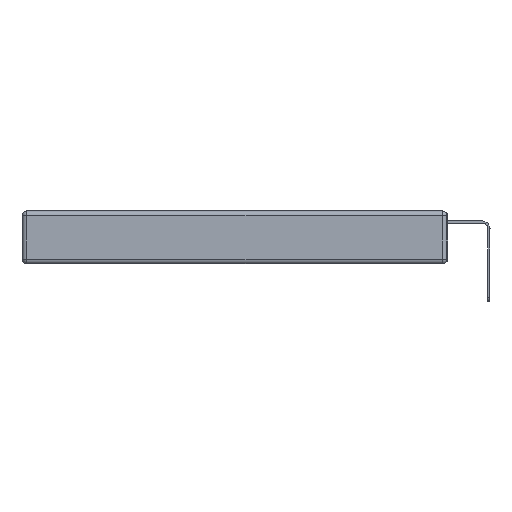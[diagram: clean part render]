
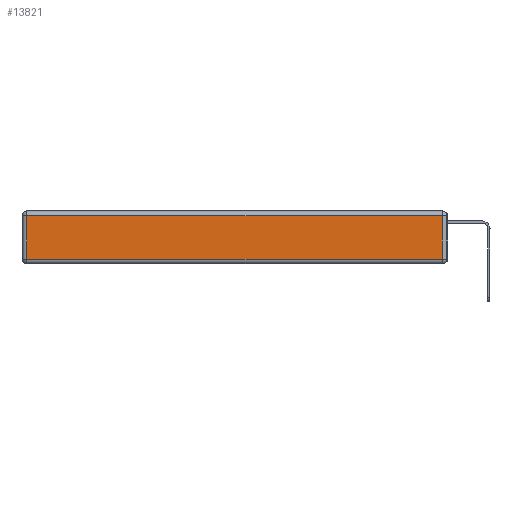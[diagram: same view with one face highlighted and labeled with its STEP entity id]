
A CAD part, left-side view. The second image highlights one B-rep face of the part: STEP entity #13821.
In plain terms, the highlighted planar face has unit normal (-1, 0, 0).
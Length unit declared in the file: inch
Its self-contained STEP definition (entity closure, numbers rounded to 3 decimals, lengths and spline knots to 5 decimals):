
#285 = CARTESIAN_POINT ( 'NONE',  ( 0., 2.72, -0.313 ) ) ;
#615 = DIRECTION ( 'NONE',  ( -1., 0., 0. ) ) ;
#757 = CARTESIAN_POINT ( 'NONE',  ( 0., 0., -0.343 ) ) ;
#773 = CARTESIAN_POINT ( 'NONE',  ( 0., 0.03, -0.03 ) ) ;
#1313 = EDGE_CURVE ( 'NONE', #16355, #19260, #4810, .T. ) ;
#2608 = LINE ( 'NONE', #7543, #11050 ) ;
#2782 = DIRECTION ( 'NONE',  ( 0., 1., 0. ) ) ;
#2871 = EDGE_LOOP ( 'NONE', ( #18262, #4706, #10884, #19595 ) ) ;
#4153 = EDGE_CURVE ( 'NONE', #19260, #10068, #19310, .T. ) ;
#4437 = CARTESIAN_POINT ( 'NONE',  ( 0., 2.72, -0.343 ) ) ;
#4706 = ORIENTED_EDGE ( 'NONE', *, *, #9290, .T. ) ;
#4810 = LINE ( 'NONE', #4437, #19940 ) ;
#7157 = CARTESIAN_POINT ( 'NONE',  ( 0., 2.72, -0.03 ) ) ;
#7543 = CARTESIAN_POINT ( 'NONE',  ( 0., 2.75, -0.03 ) ) ;
#7978 = VECTOR ( 'NONE', #19165, 39.37008 ) ;
#8050 = EDGE_CURVE ( 'NONE', #17491, #16355, #2608, .T. ) ;
#8529 = FACE_OUTER_BOUND ( 'NONE', #2871, .T. ) ;
#8962 = VECTOR ( 'NONE', #9070, 39.37008 ) ;
#9070 = DIRECTION ( 'NONE',  ( 0., 0., 1. ) ) ;
#9113 = DIRECTION ( 'NONE',  ( 0., 0., -1. ) ) ;
#9290 = EDGE_CURVE ( 'NONE', #10068, #17491, #11435, .T. ) ;
#10068 = VERTEX_POINT ( 'NONE', #13895 ) ;
#10884 = ORIENTED_EDGE ( 'NONE', *, *, #8050, .T. ) ;
#11050 = VECTOR ( 'NONE', #2782, 39.37008 ) ;
#11435 = LINE ( 'NONE', #15467, #8962 ) ;
#12833 = CARTESIAN_POINT ( 'NONE',  ( 0., 0., -0.313 ) ) ;
#13821 = ADVANCED_FACE ( 'NONE', ( #8529 ), #14880, .T. ) ;
#13895 = CARTESIAN_POINT ( 'NONE',  ( 0., 0.03, -0.313 ) ) ;
#14214 = AXIS2_PLACEMENT_3D ( 'NONE', #757, #615, #18123 ) ;
#14880 = PLANE ( 'NONE',  #14214 ) ;
#15467 = CARTESIAN_POINT ( 'NONE',  ( 0., 0.03, -0.343 ) ) ;
#16355 = VERTEX_POINT ( 'NONE', #7157 ) ;
#17491 = VERTEX_POINT ( 'NONE', #773 ) ;
#18123 = DIRECTION ( 'NONE',  ( 0., 0., 1. ) ) ;
#18262 = ORIENTED_EDGE ( 'NONE', *, *, #4153, .T. ) ;
#19165 = DIRECTION ( 'NONE',  ( 0., -1., 0. ) ) ;
#19260 = VERTEX_POINT ( 'NONE', #285 ) ;
#19310 = LINE ( 'NONE', #12833, #7978 ) ;
#19595 = ORIENTED_EDGE ( 'NONE', *, *, #1313, .T. ) ;
#19940 = VECTOR ( 'NONE', #9113, 39.37008 ) ;
